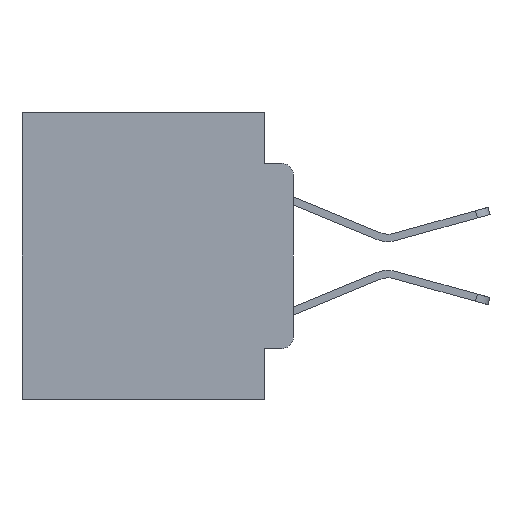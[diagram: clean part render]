
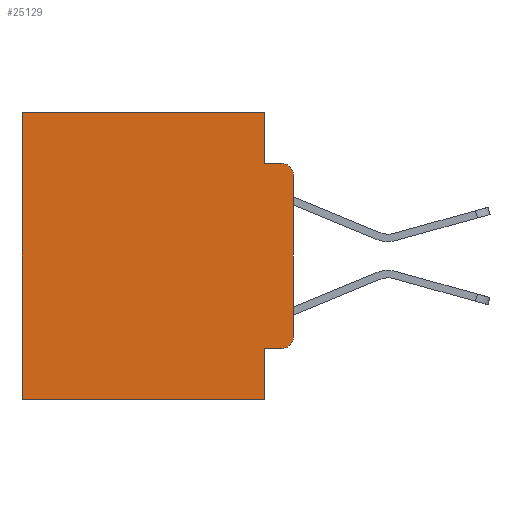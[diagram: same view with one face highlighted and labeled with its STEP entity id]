
A CAD part, left-side view. The second image highlights one B-rep face of the part: STEP entity #25129.
In plain terms, the highlighted planar face has unit normal (-1, 0, 0).
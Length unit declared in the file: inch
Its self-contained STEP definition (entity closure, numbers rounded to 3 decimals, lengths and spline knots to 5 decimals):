
#148 = AXIS2_PLACEMENT_3D ( 'NONE', #2699, #10708, #25352 ) ;
#618 = DIRECTION ( 'NONE',  ( 0., 0., -1. ) ) ;
#645 = CARTESIAN_POINT ( 'NONE',  ( 0.298, 0.051, 0. ) ) ;
#897 = AXIS2_PLACEMENT_3D ( 'NONE', #25099, #14883, #4443 ) ;
#1548 = EDGE_CURVE ( 'NONE', #7055, #2476, #7298, .T. ) ;
#2028 = CARTESIAN_POINT ( 'NONE',  ( 0.298, 0.051, -0.5 ) ) ;
#2476 = VERTEX_POINT ( 'NONE', #12509 ) ;
#2566 = CARTESIAN_POINT ( 'NONE',  ( 0.298, 0., 0. ) ) ;
#2613 = ORIENTED_EDGE ( 'NONE', *, *, #23237, .T. ) ;
#2699 = CARTESIAN_POINT ( 'NONE',  ( 0.298, 0.02, -0.1085 ) ) ;
#2727 = ORIENTED_EDGE ( 'NONE', *, *, #1548, .F. ) ;
#2782 = VECTOR ( 'NONE', #10709, 39.37008 ) ;
#4083 = DIRECTION ( 'NONE',  ( 0., 0., -1. ) ) ;
#4428 = VERTEX_POINT ( 'NONE', #25288 ) ;
#4443 = DIRECTION ( 'NONE',  ( 0., 0., -1. ) ) ;
#4728 = EDGE_LOOP ( 'NONE', ( #6200, #10939, #16724, #2727, #9876, #15951, #14753, #20497, #22254, #2613 ) ) ;
#4805 = EDGE_CURVE ( 'NONE', #20164, #4428, #20255, .T. ) ;
#5169 = AXIS2_PLACEMENT_3D ( 'NONE', #24472, #6081, #4083 ) ;
#6081 = DIRECTION ( 'NONE',  ( -1., 0., 0. ) ) ;
#6200 = ORIENTED_EDGE ( 'NONE', *, *, #13256, .F. ) ;
#6303 = LINE ( 'NONE', #14596, #14989 ) ;
#6770 = LINE ( 'NONE', #23141, #8096 ) ;
#6951 = CARTESIAN_POINT ( 'NONE',  ( 0.298, 0.473, 0. ) ) ;
#7055 = VERTEX_POINT ( 'NONE', #645 ) ;
#7298 = LINE ( 'NONE', #9299, #15398 ) ;
#7852 = CARTESIAN_POINT ( 'NONE',  ( 0.298, 0.051, -0.0885 ) ) ;
#8096 = VECTOR ( 'NONE', #618, 39.37008 ) ;
#8556 = CIRCLE ( 'NONE', #5169, 0.02 ) ;
#8648 = EDGE_CURVE ( 'NONE', #2476, #4428, #14007, .T. ) ;
#8652 = EDGE_CURVE ( 'NONE', #17142, #26285, #16035, .T. ) ;
#8876 = VECTOR ( 'NONE', #22330, 39.37008 ) ;
#8984 = LINE ( 'NONE', #17158, #12067 ) ;
#9299 = CARTESIAN_POINT ( 'NONE',  ( 0.298, 0.051, 0. ) ) ;
#9876 = ORIENTED_EDGE ( 'NONE', *, *, #25076, .T. ) ;
#10708 = DIRECTION ( 'NONE',  ( -1., 0., 0. ) ) ;
#10709 = DIRECTION ( 'NONE',  ( 0., 0., -1. ) ) ;
#10939 = ORIENTED_EDGE ( 'NONE', *, *, #4805, .T. ) ;
#11556 = DIRECTION ( 'NONE',  ( 0., 0., -1. ) ) ;
#11733 = DIRECTION ( 'NONE',  ( 0., -1., 0. ) ) ;
#11767 = EDGE_CURVE ( 'NONE', #16745, #23656, #6303, .T. ) ;
#12067 = VECTOR ( 'NONE', #15416, 39.37008 ) ;
#12509 = CARTESIAN_POINT ( 'NONE',  ( 0.298, 0.051, -0.0885 ) ) ;
#12875 = DIRECTION ( 'NONE',  ( 0., 1., 0. ) ) ;
#13256 = EDGE_CURVE ( 'NONE', #20164, #13632, #20905, .T. ) ;
#13632 = VERTEX_POINT ( 'NONE', #23038 ) ;
#14007 = LINE ( 'NONE', #7852, #23888 ) ;
#14343 = FACE_OUTER_BOUND ( 'NONE', #4728, .T. ) ;
#14596 = CARTESIAN_POINT ( 'NONE',  ( 0.298, 0., -0.5 ) ) ;
#14753 = ORIENTED_EDGE ( 'NONE', *, *, #11767, .F. ) ;
#14883 = DIRECTION ( 'NONE',  ( 1., 0., 0. ) ) ;
#14989 = VECTOR ( 'NONE', #22791, 39.37008 ) ;
#15398 = VECTOR ( 'NONE', #11556, 39.37008 ) ;
#15416 = DIRECTION ( 'NONE',  ( 0., 0., -1. ) ) ;
#15951 = ORIENTED_EDGE ( 'NONE', *, *, #25245, .T. ) ;
#16035 = LINE ( 'NONE', #24236, #8876 ) ;
#16147 = CARTESIAN_POINT ( 'NONE',  ( 0.298, 0.02, -0.4115 ) ) ;
#16724 = ORIENTED_EDGE ( 'NONE', *, *, #8648, .F. ) ;
#16745 = VERTEX_POINT ( 'NONE', #2028 ) ;
#16794 = VERTEX_POINT ( 'NONE', #6951 ) ;
#17142 = VERTEX_POINT ( 'NONE', #26383 ) ;
#17158 = CARTESIAN_POINT ( 'NONE',  ( 0.298, 0.473, 0. ) ) ;
#18534 = CARTESIAN_POINT ( 'NONE',  ( 0.298, 0., -0.1085 ) ) ;
#19048 = CARTESIAN_POINT ( 'NONE',  ( 0.298, 0., 0. ) ) ;
#20126 = CARTESIAN_POINT ( 'NONE',  ( 0.298, 0.473, -0.5 ) ) ;
#20164 = VERTEX_POINT ( 'NONE', #18534 ) ;
#20255 = CIRCLE ( 'NONE', #148, 0.02 ) ;
#20497 = ORIENTED_EDGE ( 'NONE', *, *, #22445, .F. ) ;
#20905 = LINE ( 'NONE', #2566, #2782 ) ;
#22254 = ORIENTED_EDGE ( 'NONE', *, *, #8652, .T. ) ;
#22330 = DIRECTION ( 'NONE',  ( 0., -1., 0. ) ) ;
#22445 = EDGE_CURVE ( 'NONE', #17142, #16745, #6770, .T. ) ;
#22540 = PLANE ( 'NONE',  #897 ) ;
#22791 = DIRECTION ( 'NONE',  ( 0., 1., 0. ) ) ;
#23038 = CARTESIAN_POINT ( 'NONE',  ( 0.298, 0., -0.3915 ) ) ;
#23141 = CARTESIAN_POINT ( 'NONE',  ( 0.298, 0.051, 0. ) ) ;
#23237 = EDGE_CURVE ( 'NONE', #26285, #13632, #8556, .T. ) ;
#23656 = VERTEX_POINT ( 'NONE', #20126 ) ;
#23888 = VECTOR ( 'NONE', #11733, 39.37008 ) ;
#24236 = CARTESIAN_POINT ( 'NONE',  ( 0.298, 0.051, -0.4115 ) ) ;
#24440 = VECTOR ( 'NONE', #12875, 39.37008 ) ;
#24472 = CARTESIAN_POINT ( 'NONE',  ( 0.298, 0.02, -0.3915 ) ) ;
#24567 = LINE ( 'NONE', #19048, #24440 ) ;
#25076 = EDGE_CURVE ( 'NONE', #7055, #16794, #24567, .T. ) ;
#25099 = CARTESIAN_POINT ( 'NONE',  ( 0.298, 0., 0. ) ) ;
#25129 = ADVANCED_FACE ( 'NONE', ( #14343 ), #22540, .F. ) ;
#25245 = EDGE_CURVE ( 'NONE', #16794, #23656, #8984, .T. ) ;
#25288 = CARTESIAN_POINT ( 'NONE',  ( 0.298, 0.02, -0.0885 ) ) ;
#25352 = DIRECTION ( 'NONE',  ( 0., 0., -1. ) ) ;
#26285 = VERTEX_POINT ( 'NONE', #16147 ) ;
#26383 = CARTESIAN_POINT ( 'NONE',  ( 0.298, 0.051, -0.4115 ) ) ;
